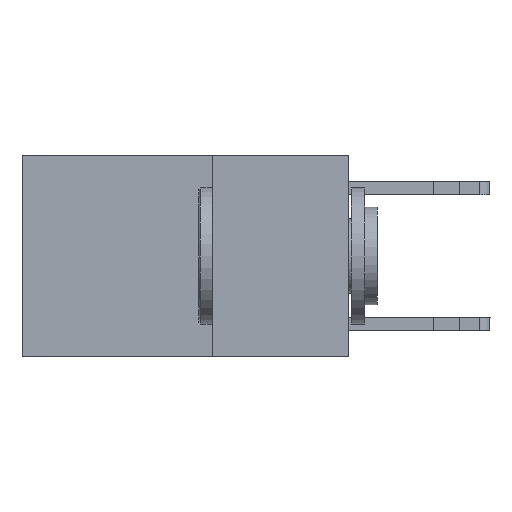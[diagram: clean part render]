
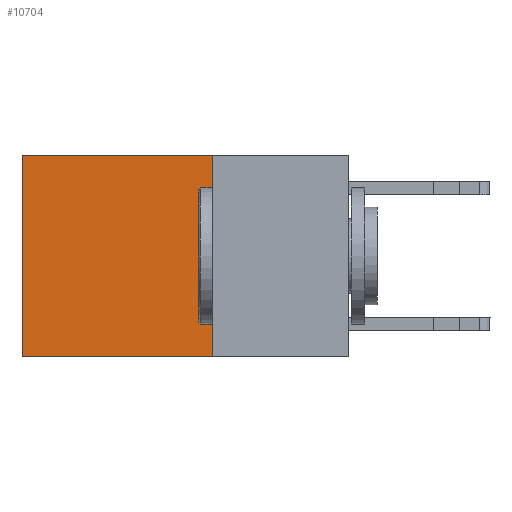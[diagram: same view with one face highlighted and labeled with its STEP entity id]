
A CAD part, left-side view. The second image highlights one B-rep face of the part: STEP entity #10704.
In plain terms, the highlighted planar face has unit normal (-1, 0, 0).
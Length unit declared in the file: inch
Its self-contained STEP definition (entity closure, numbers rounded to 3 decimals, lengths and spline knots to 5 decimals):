
#356 = CARTESIAN_POINT ( 'NONE',  ( 0.2625, 0.25, -0.37 ) ) ;
#452 = CARTESIAN_POINT ( 'NONE',  ( 0.2625, 0.25, 0. ) ) ;
#768 = LINE ( 'NONE', #452, #10557 ) ;
#962 = DIRECTION ( 'NONE',  ( 0., 0., -1. ) ) ;
#1057 = LINE ( 'NONE', #1816, #6218 ) ;
#1646 = LINE ( 'NONE', #356, #11280 ) ;
#1816 = CARTESIAN_POINT ( 'NONE',  ( 0.2625, 0.6, 0. ) ) ;
#2021 = ORIENTED_EDGE ( 'NONE', *, *, #6456, .F. ) ;
#2656 = CARTESIAN_POINT ( 'NONE',  ( 0.2625, 0.25, 0. ) ) ;
#2766 = EDGE_CURVE ( 'NONE', #4002, #3743, #768, .T. ) ;
#3228 = ORIENTED_EDGE ( 'NONE', *, *, #7233, .F. ) ;
#3743 = VERTEX_POINT ( 'NONE', #5881 ) ;
#4002 = VERTEX_POINT ( 'NONE', #4352 ) ;
#4182 = EDGE_CURVE ( 'NONE', #3743, #6343, #1057, .T. ) ;
#4352 = CARTESIAN_POINT ( 'NONE',  ( 0.2625, 0.25, 0. ) ) ;
#5520 = DIRECTION ( 'NONE',  ( 0., 0., -1. ) ) ;
#5856 = AXIS2_PLACEMENT_3D ( 'NONE', #2656, #11014, #5520 ) ;
#5858 = CARTESIAN_POINT ( 'NONE',  ( 0.2625, 0.25, 0. ) ) ;
#5878 = VECTOR ( 'NONE', #962, 39.37008 ) ;
#5881 = CARTESIAN_POINT ( 'NONE',  ( 0.2625, 0.6, 0. ) ) ;
#5941 = FACE_OUTER_BOUND ( 'NONE', #8608, .T. ) ;
#6173 = LINE ( 'NONE', #5858, #5878 ) ;
#6218 = VECTOR ( 'NONE', #8458, 39.37008 ) ;
#6247 = ORIENTED_EDGE ( 'NONE', *, *, #2766, .T. ) ;
#6343 = VERTEX_POINT ( 'NONE', #12052 ) ;
#6456 = EDGE_CURVE ( 'NONE', #4002, #9468, #6173, .T. ) ;
#7233 = EDGE_CURVE ( 'NONE', #9468, #6343, #1646, .T. ) ;
#8458 = DIRECTION ( 'NONE',  ( 0., 0., -1. ) ) ;
#8608 = EDGE_LOOP ( 'NONE', ( #10863, #3228, #2021, #6247 ) ) ;
#9032 = DIRECTION ( 'NONE',  ( 0., 1., 0. ) ) ;
#9206 = PLANE ( 'NONE',  #5856 ) ;
#9468 = VERTEX_POINT ( 'NONE', #9497 ) ;
#9497 = CARTESIAN_POINT ( 'NONE',  ( 0.2625, 0.25, -0.37 ) ) ;
#10557 = VECTOR ( 'NONE', #10932, 39.37008 ) ;
#10704 = ADVANCED_FACE ( 'NONE', ( #5941 ), #9206, .F. ) ;
#10863 = ORIENTED_EDGE ( 'NONE', *, *, #4182, .T. ) ;
#10932 = DIRECTION ( 'NONE',  ( 0., 1., 0. ) ) ;
#11014 = DIRECTION ( 'NONE',  ( 1., 0., 0. ) ) ;
#11280 = VECTOR ( 'NONE', #9032, 39.37008 ) ;
#12052 = CARTESIAN_POINT ( 'NONE',  ( 0.2625, 0.6, -0.37 ) ) ;
